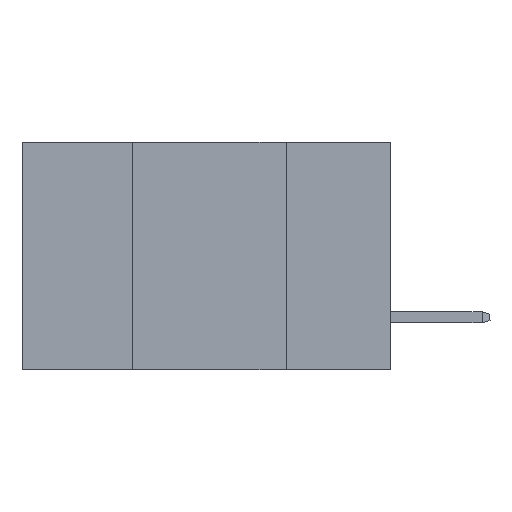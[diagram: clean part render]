
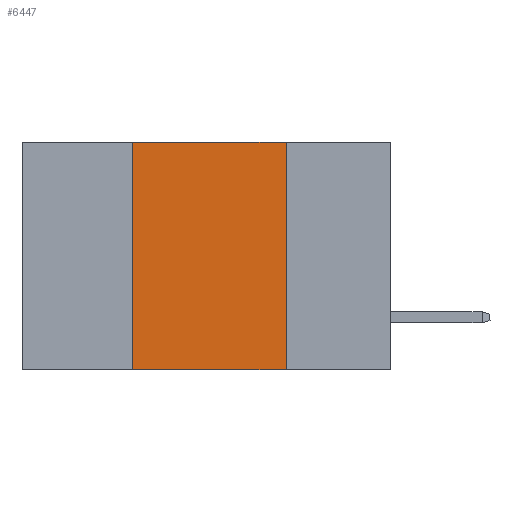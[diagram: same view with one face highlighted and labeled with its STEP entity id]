
A CAD part, left-side view. The second image highlights one B-rep face of the part: STEP entity #6447.
In plain terms, the highlighted planar face has unit normal (-1, 0, 0).
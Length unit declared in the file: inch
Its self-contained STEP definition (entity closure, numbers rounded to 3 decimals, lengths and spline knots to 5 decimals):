
#77 = VERTEX_POINT ( 'NONE', #3931 ) ;
#479 = DIRECTION ( 'NONE',  ( 0., -1., 0. ) ) ;
#525 = CARTESIAN_POINT ( 'NONE',  ( 0., 0.6, -0.37 ) ) ;
#648 = CARTESIAN_POINT ( 'NONE',  ( 0., 0.42, 0. ) ) ;
#1187 = VECTOR ( 'NONE', #10987, 39.37008 ) ;
#1467 = CARTESIAN_POINT ( 'NONE',  ( 0., 0.17, 0. ) ) ;
#1548 = EDGE_LOOP ( 'NONE', ( #12582, #10190, #6411, #3115 ) ) ;
#2449 = DIRECTION ( 'NONE',  ( 0., 0., -1. ) ) ;
#2461 = DIRECTION ( 'NONE',  ( 1., 0., 0. ) ) ;
#2463 = PLANE ( 'NONE',  #4830 ) ;
#2531 = CARTESIAN_POINT ( 'NONE',  ( 0., 0.6, 0. ) ) ;
#3115 = ORIENTED_EDGE ( 'NONE', *, *, #6633, .T. ) ;
#3710 = EDGE_CURVE ( 'NONE', #7659, #77, #11470, .T. ) ;
#3931 = CARTESIAN_POINT ( 'NONE',  ( 0., 0.17, -0.37 ) ) ;
#4830 = AXIS2_PLACEMENT_3D ( 'NONE', #2531, #2461, #2449 ) ;
#4928 = CARTESIAN_POINT ( 'NONE',  ( 0., 0.6, 0. ) ) ;
#5085 = DIRECTION ( 'NONE',  ( 0., -1., 0. ) ) ;
#6117 = VECTOR ( 'NONE', #9506, 39.37008 ) ;
#6217 = EDGE_CURVE ( 'NONE', #7153, #7659, #10517, .T. ) ;
#6362 = LINE ( 'NONE', #525, #11397 ) ;
#6411 = ORIENTED_EDGE ( 'NONE', *, *, #11094, .F. ) ;
#6447 = ADVANCED_FACE ( 'NONE', ( #11243 ), #2463, .F. ) ;
#6633 = EDGE_CURVE ( 'NONE', #12796, #77, #6362, .T. ) ;
#6768 = LINE ( 'NONE', #648, #1187 ) ;
#7049 = CARTESIAN_POINT ( 'NONE',  ( 0., 0.17, 0. ) ) ;
#7153 = VERTEX_POINT ( 'NONE', #7818 ) ;
#7659 = VERTEX_POINT ( 'NONE', #1467 ) ;
#7818 = CARTESIAN_POINT ( 'NONE',  ( 0., 0.42, 0. ) ) ;
#8502 = VECTOR ( 'NONE', #5085, 39.37008 ) ;
#9506 = DIRECTION ( 'NONE',  ( 0., 0., -1. ) ) ;
#10176 = CARTESIAN_POINT ( 'NONE',  ( 0., 0.42, -0.37 ) ) ;
#10190 = ORIENTED_EDGE ( 'NONE', *, *, #6217, .F. ) ;
#10517 = LINE ( 'NONE', #4928, #8502 ) ;
#10987 = DIRECTION ( 'NONE',  ( 0., 0., 1. ) ) ;
#11094 = EDGE_CURVE ( 'NONE', #12796, #7153, #6768, .T. ) ;
#11243 = FACE_OUTER_BOUND ( 'NONE', #1548, .T. ) ;
#11397 = VECTOR ( 'NONE', #479, 39.37008 ) ;
#11470 = LINE ( 'NONE', #7049, #6117 ) ;
#12582 = ORIENTED_EDGE ( 'NONE', *, *, #3710, .F. ) ;
#12796 = VERTEX_POINT ( 'NONE', #10176 ) ;
